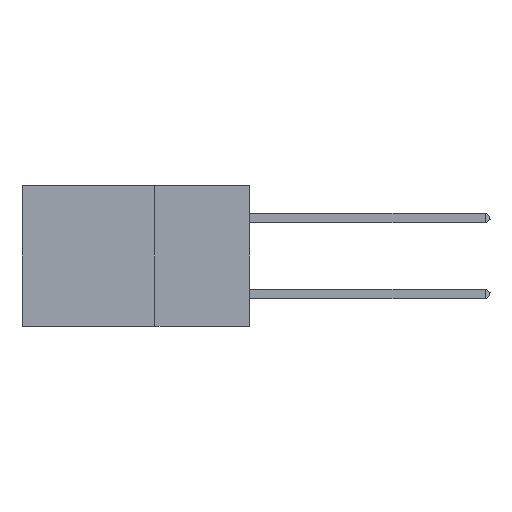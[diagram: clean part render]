
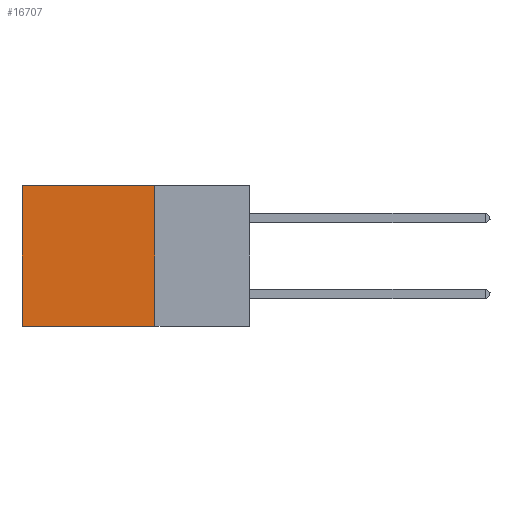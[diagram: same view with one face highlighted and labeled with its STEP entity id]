
A CAD part, left-side view. The second image highlights one B-rep face of the part: STEP entity #16707.
In plain terms, the highlighted planar face has unit normal (-1, 0, 0).
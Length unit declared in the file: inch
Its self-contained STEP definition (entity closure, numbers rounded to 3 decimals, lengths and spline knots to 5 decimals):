
#466 = ORIENTED_EDGE ( 'NONE', *, *, #37769, .T. ) ;
#5066 = ORIENTED_EDGE ( 'NONE', *, *, #22826, .T. ) ;
#5624 = DIRECTION ( 'NONE',  ( 0., 0., -1. ) ) ;
#5731 = LINE ( 'NONE', #33499, #19682 ) ;
#9725 = EDGE_CURVE ( 'NONE', #10111, #35955, #29794, .T. ) ;
#10111 = VERTEX_POINT ( 'NONE', #25426 ) ;
#10738 = VECTOR ( 'NONE', #27711, 39.37008 ) ;
#11755 = AXIS2_PLACEMENT_3D ( 'NONE', #29154, #23359, #5624 ) ;
#13079 = CARTESIAN_POINT ( 'NONE',  ( 0.2875, 0.25, 0. ) ) ;
#14047 = ORIENTED_EDGE ( 'NONE', *, *, #32020, .F. ) ;
#16503 = VERTEX_POINT ( 'NONE', #31345 ) ;
#16707 = ADVANCED_FACE ( 'NONE', ( #27580 ), #20440, .F. ) ;
#17392 = CARTESIAN_POINT ( 'NONE',  ( 0.2875, 0.25, -0.37 ) ) ;
#19682 = VECTOR ( 'NONE', #24795, 39.37008 ) ;
#20440 = PLANE ( 'NONE',  #11755 ) ;
#20628 = DIRECTION ( 'NONE',  ( 0., 1., 0. ) ) ;
#21988 = VECTOR ( 'NONE', #29040, 39.37008 ) ;
#22826 = EDGE_CURVE ( 'NONE', #29861, #35955, #5731, .T. ) ;
#23359 = DIRECTION ( 'NONE',  ( 1., 0., 0. ) ) ;
#24795 = DIRECTION ( 'NONE',  ( 0., 0., -1. ) ) ;
#25426 = CARTESIAN_POINT ( 'NONE',  ( 0.2875, 0.25, -0.37 ) ) ;
#27580 = FACE_OUTER_BOUND ( 'NONE', #29224, .T. ) ;
#27711 = DIRECTION ( 'NONE',  ( 0., 0., -1. ) ) ;
#28001 = VECTOR ( 'NONE', #20628, 39.37008 ) ;
#28230 = LINE ( 'NONE', #13079, #10738 ) ;
#28667 = CARTESIAN_POINT ( 'NONE',  ( 0.2875, 0.6, 0. ) ) ;
#29040 = DIRECTION ( 'NONE',  ( 0., 1., 0. ) ) ;
#29154 = CARTESIAN_POINT ( 'NONE',  ( 0.2875, 0.25, 0. ) ) ;
#29224 = EDGE_LOOP ( 'NONE', ( #5066, #32764, #14047, #466 ) ) ;
#29794 = LINE ( 'NONE', #17392, #21988 ) ;
#29844 = LINE ( 'NONE', #35271, #28001 ) ;
#29861 = VERTEX_POINT ( 'NONE', #28667 ) ;
#30781 = CARTESIAN_POINT ( 'NONE',  ( 0.2875, 0.6, -0.37 ) ) ;
#31345 = CARTESIAN_POINT ( 'NONE',  ( 0.2875, 0.25, 0. ) ) ;
#32020 = EDGE_CURVE ( 'NONE', #16503, #10111, #28230, .T. ) ;
#32764 = ORIENTED_EDGE ( 'NONE', *, *, #9725, .F. ) ;
#33499 = CARTESIAN_POINT ( 'NONE',  ( 0.2875, 0.6, 0. ) ) ;
#35271 = CARTESIAN_POINT ( 'NONE',  ( 0.2875, 0.25, 0. ) ) ;
#35955 = VERTEX_POINT ( 'NONE', #30781 ) ;
#37769 = EDGE_CURVE ( 'NONE', #16503, #29861, #29844, .T. ) ;
